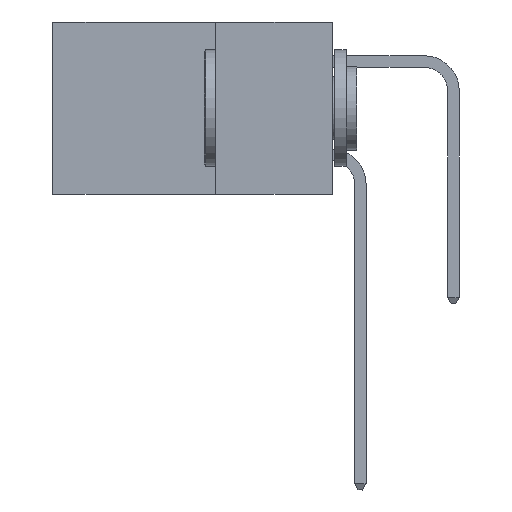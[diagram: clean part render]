
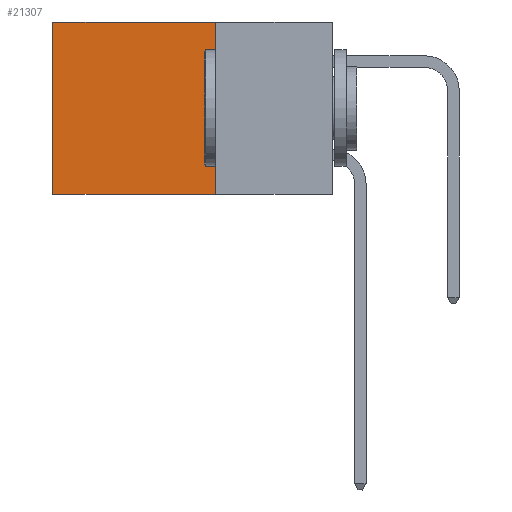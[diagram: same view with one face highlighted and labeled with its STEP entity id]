
A CAD part, left-side view. The second image highlights one B-rep face of the part: STEP entity #21307.
In plain terms, the highlighted planar face has unit normal (-1, 0, 0).
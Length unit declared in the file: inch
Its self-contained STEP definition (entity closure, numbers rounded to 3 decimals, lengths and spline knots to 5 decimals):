
#559 = VERTEX_POINT ( 'NONE', #20879 ) ;
#600 = CARTESIAN_POINT ( 'NONE',  ( 0.298, 0.25, 0. ) ) ;
#1534 = EDGE_CURVE ( 'NONE', #13443, #559, #13402, .T. ) ;
#3035 = DIRECTION ( 'NONE',  ( 0., 0., -1. ) ) ;
#3300 = CARTESIAN_POINT ( 'NONE',  ( 0.298, 0.6, 0. ) ) ;
#3986 = ORIENTED_EDGE ( 'NONE', *, *, #1534, .F. ) ;
#4113 = DIRECTION ( 'NONE',  ( 1., 0., 0. ) ) ;
#4700 = CARTESIAN_POINT ( 'NONE',  ( 0.298, 0.25, -0.37 ) ) ;
#5004 = LINE ( 'NONE', #13613, #15751 ) ;
#5504 = EDGE_CURVE ( 'NONE', #11681, #22013, #5004, .T. ) ;
#6166 = LINE ( 'NONE', #9940, #18468 ) ;
#6976 = FACE_OUTER_BOUND ( 'NONE', #10885, .T. ) ;
#8146 = DIRECTION ( 'NONE',  ( 0., 0., -1. ) ) ;
#8462 = CARTESIAN_POINT ( 'NONE',  ( 0.298, 0.25, -0.37 ) ) ;
#9416 = CARTESIAN_POINT ( 'NONE',  ( 0.298, 0.25, 0. ) ) ;
#9940 = CARTESIAN_POINT ( 'NONE',  ( 0.298, 0.25, 0. ) ) ;
#10037 = DIRECTION ( 'NONE',  ( 0., 1., 0. ) ) ;
#10058 = AXIS2_PLACEMENT_3D ( 'NONE', #600, #4113, #12507 ) ;
#10460 = ORIENTED_EDGE ( 'NONE', *, *, #5504, .T. ) ;
#10805 = PLANE ( 'NONE',  #10058 ) ;
#10885 = EDGE_LOOP ( 'NONE', ( #14898, #3986, #15983, #10460 ) ) ;
#11681 = VERTEX_POINT ( 'NONE', #9416 ) ;
#12507 = DIRECTION ( 'NONE',  ( 0., 0., -1. ) ) ;
#13402 = LINE ( 'NONE', #8462, #16086 ) ;
#13443 = VERTEX_POINT ( 'NONE', #4700 ) ;
#13480 = CARTESIAN_POINT ( 'NONE',  ( 0.298, 0.6, 0. ) ) ;
#13613 = CARTESIAN_POINT ( 'NONE',  ( 0.298, 0.25, 0. ) ) ;
#14385 = EDGE_CURVE ( 'NONE', #22013, #559, #16764, .T. ) ;
#14898 = ORIENTED_EDGE ( 'NONE', *, *, #14385, .T. ) ;
#15751 = VECTOR ( 'NONE', #10037, 39.37008 ) ;
#15983 = ORIENTED_EDGE ( 'NONE', *, *, #16274, .F. ) ;
#16086 = VECTOR ( 'NONE', #18534, 39.37008 ) ;
#16274 = EDGE_CURVE ( 'NONE', #11681, #13443, #6166, .T. ) ;
#16764 = LINE ( 'NONE', #13480, #20776 ) ;
#18468 = VECTOR ( 'NONE', #3035, 39.37008 ) ;
#18534 = DIRECTION ( 'NONE',  ( 0., 1., 0. ) ) ;
#20776 = VECTOR ( 'NONE', #8146, 39.37008 ) ;
#20879 = CARTESIAN_POINT ( 'NONE',  ( 0.298, 0.6, -0.37 ) ) ;
#21307 = ADVANCED_FACE ( 'NONE', ( #6976 ), #10805, .F. ) ;
#22013 = VERTEX_POINT ( 'NONE', #3300 ) ;
